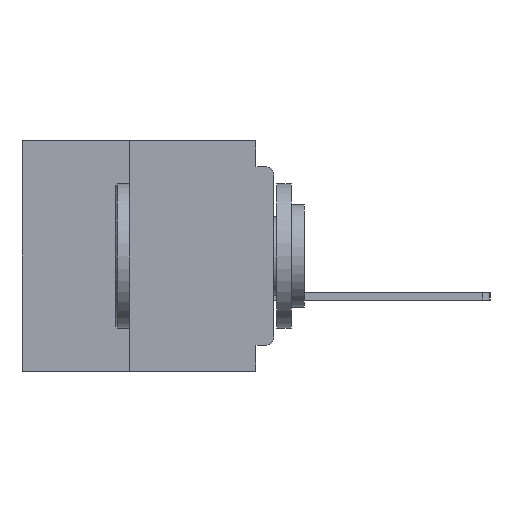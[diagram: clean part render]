
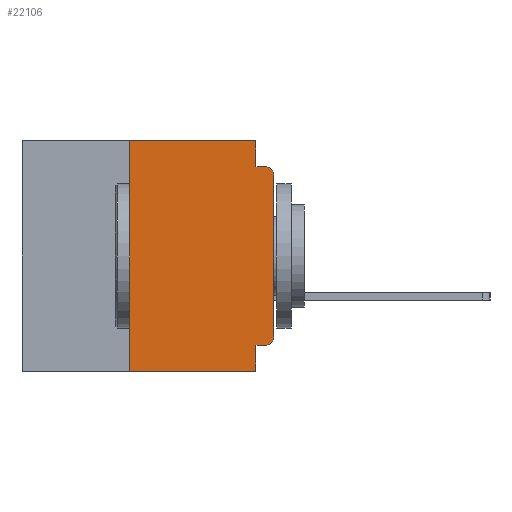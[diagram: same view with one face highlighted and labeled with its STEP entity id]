
A CAD part, left-side view. The second image highlights one B-rep face of the part: STEP entity #22106.
In plain terms, the highlighted planar face has unit normal (-1, 0, 0).
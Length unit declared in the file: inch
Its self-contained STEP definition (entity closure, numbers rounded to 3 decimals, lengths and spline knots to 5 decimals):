
#1460 = CARTESIAN_POINT ( 'NONE',  ( 0., 0.25, -0.4 ) ) ;
#1468 = ORIENTED_EDGE ( 'NONE', *, *, #32230, .F. ) ;
#2079 = EDGE_CURVE ( 'NONE', #32001, #46320, #17226, .T. ) ;
#2206 = EDGE_LOOP ( 'NONE', ( #29630, #14063, #43783, #1468, #12197, #8715, #41908, #8213, #22727, #42802 ) ) ;
#3183 = DIRECTION ( 'NONE',  ( 1., 0., 0. ) ) ;
#3605 = CARTESIAN_POINT ( 'NONE',  ( 0., 0., -0.355 ) ) ;
#4163 = CARTESIAN_POINT ( 'NONE',  ( 0., 0.25, 0. ) ) ;
#5097 = DIRECTION ( 'NONE',  ( 0., -1., 0. ) ) ;
#5814 = LINE ( 'NONE', #16213, #44279 ) ;
#6889 = EDGE_CURVE ( 'NONE', #38623, #46320, #26322, .T. ) ;
#8020 = VERTEX_POINT ( 'NONE', #47256 ) ;
#8213 = ORIENTED_EDGE ( 'NONE', *, *, #44100, .F. ) ;
#8715 = ORIENTED_EDGE ( 'NONE', *, *, #27034, .F. ) ;
#9920 = CARTESIAN_POINT ( 'NONE',  ( 0., 0.031, 0. ) ) ;
#10607 = DIRECTION ( 'NONE',  ( -1., 0., 0. ) ) ;
#10944 = DIRECTION ( 'NONE',  ( -1., 0., 0. ) ) ;
#11009 = VECTOR ( 'NONE', #18712, 39.37008 ) ;
#11319 = CIRCLE ( 'NONE', #17682, 0.015 ) ;
#11950 = VECTOR ( 'NONE', #39596, 39.37008 ) ;
#12197 = ORIENTED_EDGE ( 'NONE', *, *, #23241, .F. ) ;
#13596 = CARTESIAN_POINT ( 'NONE',  ( 0., 0., 0. ) ) ;
#13954 = VERTEX_POINT ( 'NONE', #4163 ) ;
#14063 = ORIENTED_EDGE ( 'NONE', *, *, #6889, .T. ) ;
#14256 = VERTEX_POINT ( 'NONE', #9920 ) ;
#14448 = EDGE_CURVE ( 'NONE', #38744, #24483, #17402, .T. ) ;
#16213 = CARTESIAN_POINT ( 'NONE',  ( 0., 0.437, -0.4 ) ) ;
#17226 = LINE ( 'NONE', #35706, #45727 ) ;
#17402 = LINE ( 'NONE', #3605, #45915 ) ;
#17521 = CARTESIAN_POINT ( 'NONE',  ( 0., 0.437, 0. ) ) ;
#17682 = AXIS2_PLACEMENT_3D ( 'NONE', #32823, #10607, #36605 ) ;
#18712 = DIRECTION ( 'NONE',  ( 0., 0., -1. ) ) ;
#19368 = VERTEX_POINT ( 'NONE', #31411 ) ;
#20728 = VERTEX_POINT ( 'NONE', #1460 ) ;
#21822 = PLANE ( 'NONE',  #27745 ) ;
#22028 = LINE ( 'NONE', #44741, #11009 ) ;
#22106 = ADVANCED_FACE ( 'NONE', ( #38635 ), #21822, .F. ) ;
#22727 = ORIENTED_EDGE ( 'NONE', *, *, #14448, .F. ) ;
#23241 = EDGE_CURVE ( 'NONE', #13954, #14256, #44367, .T. ) ;
#23590 = CARTESIAN_POINT ( 'NONE',  ( 0., 0.25, -0.4 ) ) ;
#24483 = VERTEX_POINT ( 'NONE', #35164 ) ;
#24786 = CARTESIAN_POINT ( 'NONE',  ( 0., 0.015, -0.355 ) ) ;
#25045 = VECTOR ( 'NONE', #33261, 39.37008 ) ;
#25960 = DIRECTION ( 'NONE',  ( 0., 1., 0. ) ) ;
#26322 = CIRCLE ( 'NONE', #32950, 0.015 ) ;
#27034 = EDGE_CURVE ( 'NONE', #20728, #13954, #43938, .T. ) ;
#27327 = EDGE_CURVE ( 'NONE', #38744, #19368, #11319, .T. ) ;
#27350 = DIRECTION ( 'NONE',  ( 0., 0., 1. ) ) ;
#27745 = AXIS2_PLACEMENT_3D ( 'NONE', #47847, #3183, #29305 ) ;
#29148 = CARTESIAN_POINT ( 'NONE',  ( 0., 0.015, -0.045 ) ) ;
#29305 = DIRECTION ( 'NONE',  ( 0., 0., -1. ) ) ;
#29630 = ORIENTED_EDGE ( 'NONE', *, *, #40886, .T. ) ;
#31411 = CARTESIAN_POINT ( 'NONE',  ( 0., 0., -0.34 ) ) ;
#31686 = LINE ( 'NONE', #13596, #11950 ) ;
#32001 = VERTEX_POINT ( 'NONE', #35783 ) ;
#32230 = EDGE_CURVE ( 'NONE', #14256, #32001, #22028, .T. ) ;
#32267 = DIRECTION ( 'NONE',  ( 0., -1., 0. ) ) ;
#32823 = CARTESIAN_POINT ( 'NONE',  ( 0., 0.015, -0.34 ) ) ;
#32950 = AXIS2_PLACEMENT_3D ( 'NONE', #33170, #10944, #36949 ) ;
#33170 = CARTESIAN_POINT ( 'NONE',  ( 0., 0.015, -0.06 ) ) ;
#33261 = DIRECTION ( 'NONE',  ( 0., 0., -1. ) ) ;
#35164 = CARTESIAN_POINT ( 'NONE',  ( 0., 0.031, -0.355 ) ) ;
#35706 = CARTESIAN_POINT ( 'NONE',  ( 0., 0., -0.045 ) ) ;
#35783 = CARTESIAN_POINT ( 'NONE',  ( 0., 0.031, -0.045 ) ) ;
#35916 = DIRECTION ( 'NONE',  ( 0., -1., 0. ) ) ;
#36605 = DIRECTION ( 'NONE',  ( 0., 0., -1. ) ) ;
#36949 = DIRECTION ( 'NONE',  ( 0., 0., -1. ) ) ;
#37035 = CARTESIAN_POINT ( 'NONE',  ( 0., 0.031, -0.4 ) ) ;
#38623 = VERTEX_POINT ( 'NONE', #46313 ) ;
#38635 = FACE_OUTER_BOUND ( 'NONE', #2206, .T. ) ;
#38744 = VERTEX_POINT ( 'NONE', #24786 ) ;
#39596 = DIRECTION ( 'NONE',  ( 0., 0., 1. ) ) ;
#40886 = EDGE_CURVE ( 'NONE', #19368, #38623, #31686, .T. ) ;
#41908 = ORIENTED_EDGE ( 'NONE', *, *, #44329, .T. ) ;
#42778 = VECTOR ( 'NONE', #27350, 39.37008 ) ;
#42802 = ORIENTED_EDGE ( 'NONE', *, *, #27327, .T. ) ;
#43783 = ORIENTED_EDGE ( 'NONE', *, *, #2079, .F. ) ;
#43938 = LINE ( 'NONE', #23590, #42778 ) ;
#44100 = EDGE_CURVE ( 'NONE', #24483, #8020, #44876, .T. ) ;
#44279 = VECTOR ( 'NONE', #5097, 39.37008 ) ;
#44329 = EDGE_CURVE ( 'NONE', #20728, #8020, #5814, .T. ) ;
#44367 = LINE ( 'NONE', #17521, #47823 ) ;
#44741 = CARTESIAN_POINT ( 'NONE',  ( 0., 0.031, 0. ) ) ;
#44876 = LINE ( 'NONE', #37035, #25045 ) ;
#45727 = VECTOR ( 'NONE', #35916, 39.37008 ) ;
#45915 = VECTOR ( 'NONE', #25960, 39.37008 ) ;
#46313 = CARTESIAN_POINT ( 'NONE',  ( 0., 0., -0.06 ) ) ;
#46320 = VERTEX_POINT ( 'NONE', #29148 ) ;
#47256 = CARTESIAN_POINT ( 'NONE',  ( 0., 0.031, -0.4 ) ) ;
#47823 = VECTOR ( 'NONE', #32267, 39.37008 ) ;
#47847 = CARTESIAN_POINT ( 'NONE',  ( 0., 0.437, 0. ) ) ;
